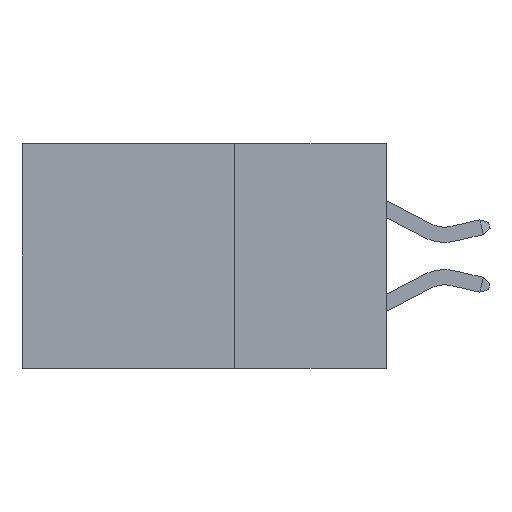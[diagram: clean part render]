
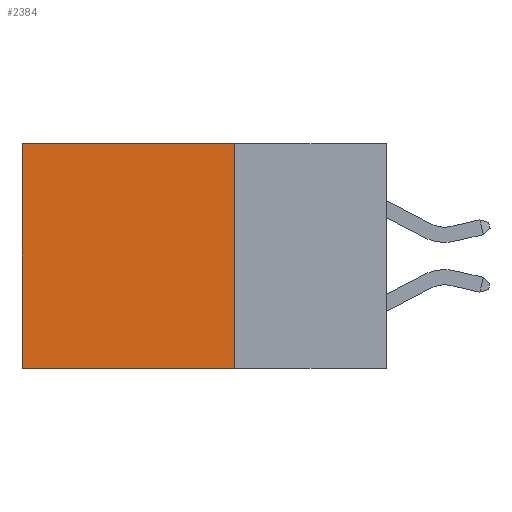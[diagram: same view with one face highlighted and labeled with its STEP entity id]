
A CAD part, left-side view. The second image highlights one B-rep face of the part: STEP entity #2384.
In plain terms, the highlighted planar face has unit normal (-1, 0, 0).
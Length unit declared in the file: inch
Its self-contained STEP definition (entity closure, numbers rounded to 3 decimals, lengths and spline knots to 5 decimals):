
#132 = VERTEX_POINT ( 'NONE', #8506 ) ;
#2093 = ORIENTED_EDGE ( 'NONE', *, *, #5383, .F. ) ;
#2196 = LINE ( 'NONE', #6578, #5214 ) ;
#2384 = ADVANCED_FACE ( 'NONE', ( #6039 ), #7299, .F. ) ;
#2779 = VERTEX_POINT ( 'NONE', #9559 ) ;
#3207 = VERTEX_POINT ( 'NONE', #6607 ) ;
#3260 = EDGE_CURVE ( 'NONE', #3207, #132, #12606, .T. ) ;
#3393 = CARTESIAN_POINT ( 'NONE',  ( 0.298, 0.25, 0. ) ) ;
#3901 = CARTESIAN_POINT ( 'NONE',  ( 0.298, 0.25, -0.37 ) ) ;
#4700 = LINE ( 'NONE', #3393, #7362 ) ;
#5214 = VECTOR ( 'NONE', #12296, 39.37008 ) ;
#5237 = VECTOR ( 'NONE', #12260, 39.37008 ) ;
#5383 = EDGE_CURVE ( 'NONE', #3207, #6548, #4700, .T. ) ;
#6039 = FACE_OUTER_BOUND ( 'NONE', #7978, .T. ) ;
#6548 = VERTEX_POINT ( 'NONE', #7562 ) ;
#6578 = CARTESIAN_POINT ( 'NONE',  ( 0.298, 0.6, 0. ) ) ;
#6607 = CARTESIAN_POINT ( 'NONE',  ( 0.298, 0.25, 0. ) ) ;
#6648 = VECTOR ( 'NONE', #12610, 39.37008 ) ;
#6650 = DIRECTION ( 'NONE',  ( 0., 0., -1. ) ) ;
#7299 = PLANE ( 'NONE',  #11732 ) ;
#7362 = VECTOR ( 'NONE', #6650, 39.37008 ) ;
#7562 = CARTESIAN_POINT ( 'NONE',  ( 0.298, 0.25, -0.37 ) ) ;
#7931 = ORIENTED_EDGE ( 'NONE', *, *, #9069, .F. ) ;
#7938 = DIRECTION ( 'NONE',  ( 0., 0., -1. ) ) ;
#7978 = EDGE_LOOP ( 'NONE', ( #10363, #7931, #2093, #8243 ) ) ;
#8243 = ORIENTED_EDGE ( 'NONE', *, *, #3260, .T. ) ;
#8506 = CARTESIAN_POINT ( 'NONE',  ( 0.298, 0.6, 0. ) ) ;
#8595 = DIRECTION ( 'NONE',  ( 1., 0., 0. ) ) ;
#8756 = CARTESIAN_POINT ( 'NONE',  ( 0.298, 0.25, 0. ) ) ;
#9069 = EDGE_CURVE ( 'NONE', #6548, #2779, #9831, .T. ) ;
#9545 = EDGE_CURVE ( 'NONE', #132, #2779, #2196, .T. ) ;
#9559 = CARTESIAN_POINT ( 'NONE',  ( 0.298, 0.6, -0.37 ) ) ;
#9831 = LINE ( 'NONE', #3901, #6648 ) ;
#10363 = ORIENTED_EDGE ( 'NONE', *, *, #9545, .T. ) ;
#11732 = AXIS2_PLACEMENT_3D ( 'NONE', #8756, #8595, #7938 ) ;
#12055 = CARTESIAN_POINT ( 'NONE',  ( 0.298, 0.25, 0. ) ) ;
#12260 = DIRECTION ( 'NONE',  ( 0., 1., 0. ) ) ;
#12296 = DIRECTION ( 'NONE',  ( 0., 0., -1. ) ) ;
#12606 = LINE ( 'NONE', #12055, #5237 ) ;
#12610 = DIRECTION ( 'NONE',  ( 0., 1., 0. ) ) ;
